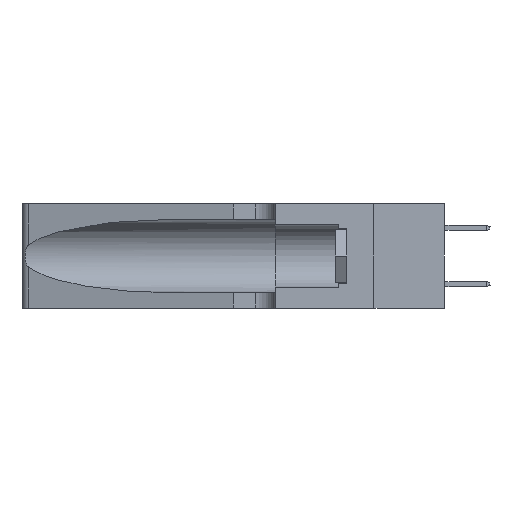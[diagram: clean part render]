
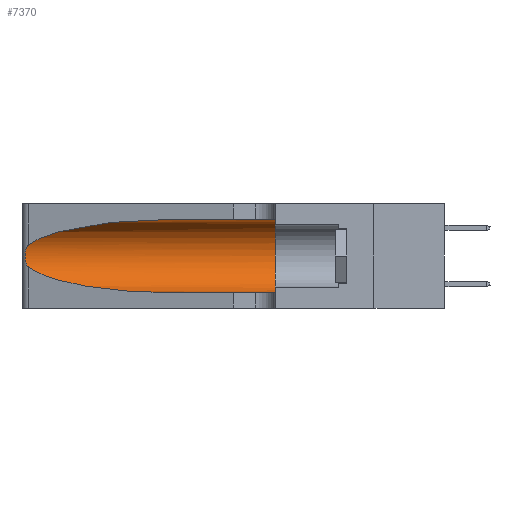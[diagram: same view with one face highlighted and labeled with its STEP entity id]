
A CAD part, left-side view. The second image highlights one B-rep face of the part: STEP entity #7370.
In plain terms, the highlighted cylindrical face has radius 3.308 mm (diameter 6.617 mm), a partial arc.
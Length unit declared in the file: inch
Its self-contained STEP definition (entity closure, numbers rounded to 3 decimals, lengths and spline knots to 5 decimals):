
#31 =( BOUNDED_CURVE ( )  B_SPLINE_CURVE ( 3, ( #3100, #19999, #18044, #6822 ),
 .UNSPECIFIED., .F., .F. ) 
 B_SPLINE_CURVE_WITH_KNOTS ( ( 4, 4 ),
 ( 3.44316, 4.71239 ),
 .UNSPECIFIED. ) 
 CURVE ( )  GEOMETRIC_REPRESENTATION_ITEM ( )  RATIONAL_B_SPLINE_CURVE ( ( 1., 0.87, 0.87, 1. ) ) 
 REPRESENTATION_ITEM ( '' )  );
#126 = DIRECTION ( 'NONE',  ( 0., 0., 1. ) ) ;
#391 = ORIENTED_EDGE ( 'NONE', *, *, #3345, .T. ) ;
#1098 = CARTESIAN_POINT ( 'NONE',  ( 0.1305, 0.72297, 0.31525 ) ) ;
#1652 = ORIENTED_EDGE ( 'NONE', *, *, #15812, .T. ) ;
#1826 = CARTESIAN_POINT ( 'NONE',  ( 0.25555, 1.22994, 0.2215 ) ) ;
#1830 = B_SPLINE_CURVE_WITH_KNOTS ( 'NONE', 3,
 ( #14915, #1826, #14833, #22436, #9628, #18880, #13125, #1988, #5570, #18568, #7405, #20450, #11188, #13044 ),
 .UNSPECIFIED., .F., .F.,
 ( 4, 2, 2, 2, 2, 2, 4 ),
 ( 0., 0.00027, 0.00053, 0.00107, 0.0016, 0.00187, 0.00214 ),
 .UNSPECIFIED. ) ;
#1988 = CARTESIAN_POINT ( 'NONE',  ( 0.26075, 1.23896, 0.178 ) ) ;
#2034 = ORIENTED_EDGE ( 'NONE', *, *, #16532, .T. ) ;
#2624 = ORIENTED_EDGE ( 'NONE', *, *, #9423, .T. ) ;
#2818 = ORIENTED_EDGE ( 'NONE', *, *, #18243, .F. ) ;
#3100 = CARTESIAN_POINT ( 'NONE',  ( 0.25487, 1.22718, 0.14631 ) ) ;
#3345 = EDGE_CURVE ( 'NONE', #7866, #5261, #1830, .T. ) ;
#4031 = CIRCLE ( 'NONE', #21545, 0.13025 ) ;
#4143 = CARTESIAN_POINT ( 'NONE',  ( 0.1305, 1.61858, 0.31525 ) ) ;
#4534 = CARTESIAN_POINT ( 'NONE',  ( 0.25487, 1.22718, 0.22369 ) ) ;
#4816 = EDGE_CURVE ( 'NONE', #11257, #6297, #9986, .T. ) ;
#5261 = VERTEX_POINT ( 'NONE', #15257 ) ;
#5570 = CARTESIAN_POINT ( 'NONE',  ( 0.26017, 1.23833, 0.17102 ) ) ;
#5631 = VECTOR ( 'NONE', #19195, 39.37008 ) ;
#6076 = ORIENTED_EDGE ( 'NONE', *, *, #4816, .F. ) ;
#6297 = VERTEX_POINT ( 'NONE', #12769 ) ;
#6822 = CARTESIAN_POINT ( 'NONE',  ( 0.1305, 0.72297, 0.05475 ) ) ;
#6926 = CYLINDRICAL_SURFACE ( 'NONE', #18224, 0.13025 ) ;
#7254 = CARTESIAN_POINT ( 'NONE',  ( 0.2373, 1.15595, 0.28018 ) ) ;
#7370 = ADVANCED_FACE ( 'NONE', ( #19738 ), #6926, .F. ) ;
#7405 = CARTESIAN_POINT ( 'NONE',  ( 0.25789, 1.23486, 0.15765 ) ) ;
#7866 = VERTEX_POINT ( 'NONE', #4534 ) ;
#8634 = VERTEX_POINT ( 'NONE', #11253 ) ;
#8695 =( BOUNDED_CURVE ( )  B_SPLINE_CURVE ( 3, ( #21971, #8843, #7254, #14521 ),
 .UNSPECIFIED., .F., .T. ) 
 B_SPLINE_CURVE_WITH_KNOTS ( ( 4, 4 ),
 ( 1.5708, 2.84003 ),
 .UNSPECIFIED. ) 
 CURVE ( )  GEOMETRIC_REPRESENTATION_ITEM ( )  RATIONAL_B_SPLINE_CURVE ( ( 1., 0.87, 0.87, 1. ) ) 
 REPRESENTATION_ITEM ( '' )  );
#8745 = CARTESIAN_POINT ( 'NONE',  ( 0.1305, 0.35, 0.185 ) ) ;
#8843 = CARTESIAN_POINT ( 'NONE',  ( 0.18966, 0.96281, 0.31525 ) ) ;
#8918 = LINE ( 'NONE', #20471, #18461 ) ;
#9423 = EDGE_CURVE ( 'NONE', #11257, #7866, #8695, .T. ) ;
#9628 = CARTESIAN_POINT ( 'NONE',  ( 0.25854, 1.2359, 0.20912 ) ) ;
#9986 = LINE ( 'NONE', #4143, #5631 ) ;
#11188 = CARTESIAN_POINT ( 'NONE',  ( 0.25555, 1.22993, 0.14849 ) ) ;
#11253 = CARTESIAN_POINT ( 'NONE',  ( 0.1305, 0.72297, 0.05475 ) ) ;
#11257 = VERTEX_POINT ( 'NONE', #1098 ) ;
#11430 = DIRECTION ( 'NONE',  ( 0., 0., -1. ) ) ;
#12769 = CARTESIAN_POINT ( 'NONE',  ( 0.1305, 0.35, 0.31525 ) ) ;
#13040 = CARTESIAN_POINT ( 'NONE',  ( 0.1305, 0.35, 0.05475 ) ) ;
#13044 = CARTESIAN_POINT ( 'NONE',  ( 0.25487, 1.22718, 0.14631 ) ) ;
#13125 = CARTESIAN_POINT ( 'NONE',  ( 0.26075, 1.23896, 0.19203 ) ) ;
#14042 = EDGE_LOOP ( 'NONE', ( #2624, #391, #1652, #2034, #2818, #6076 ) ) ;
#14521 = CARTESIAN_POINT ( 'NONE',  ( 0.25487, 1.22718, 0.22369 ) ) ;
#14833 = CARTESIAN_POINT ( 'NONE',  ( 0.25639, 1.23184, 0.21858 ) ) ;
#14915 = CARTESIAN_POINT ( 'NONE',  ( 0.25487, 1.22718, 0.22369 ) ) ;
#15257 = CARTESIAN_POINT ( 'NONE',  ( 0.25487, 1.22718, 0.14631 ) ) ;
#15812 = EDGE_CURVE ( 'NONE', #5261, #8634, #31, .T. ) ;
#16091 = VERTEX_POINT ( 'NONE', #13040 ) ;
#16483 = DIRECTION ( 'NONE',  ( 0., -1., 0. ) ) ;
#16532 = EDGE_CURVE ( 'NONE', #8634, #16091, #8918, .T. ) ;
#18044 = CARTESIAN_POINT ( 'NONE',  ( 0.18966, 0.96281, 0.05475 ) ) ;
#18224 = AXIS2_PLACEMENT_3D ( 'NONE', #21925, #23648, #11430 ) ;
#18243 = EDGE_CURVE ( 'NONE', #6297, #16091, #4031, .T. ) ;
#18461 = VECTOR ( 'NONE', #16483, 39.37008 ) ;
#18568 = CARTESIAN_POINT ( 'NONE',  ( 0.25856, 1.23593, 0.16098 ) ) ;
#18880 = CARTESIAN_POINT ( 'NONE',  ( 0.26018, 1.23835, 0.19895 ) ) ;
#19195 = DIRECTION ( 'NONE',  ( 0., -1., 0. ) ) ;
#19738 = FACE_OUTER_BOUND ( 'NONE', #14042, .T. ) ;
#19999 = CARTESIAN_POINT ( 'NONE',  ( 0.2373, 1.15595, 0.08982 ) ) ;
#20450 = CARTESIAN_POINT ( 'NONE',  ( 0.25639, 1.23186, 0.15144 ) ) ;
#20471 = CARTESIAN_POINT ( 'NONE',  ( 0.1305, 1.61858, 0.05475 ) ) ;
#21545 = AXIS2_PLACEMENT_3D ( 'NONE', #8745, #23754, #126 ) ;
#21925 = CARTESIAN_POINT ( 'NONE',  ( 0.1305, 1.61858, 0.185 ) ) ;
#21971 = CARTESIAN_POINT ( 'NONE',  ( 0.1305, 0.72297, 0.31525 ) ) ;
#22436 = CARTESIAN_POINT ( 'NONE',  ( 0.25787, 1.23484, 0.2124 ) ) ;
#23648 = DIRECTION ( 'NONE',  ( 0., -1., 0. ) ) ;
#23754 = DIRECTION ( 'NONE',  ( 0., 1., 0. ) ) ;
